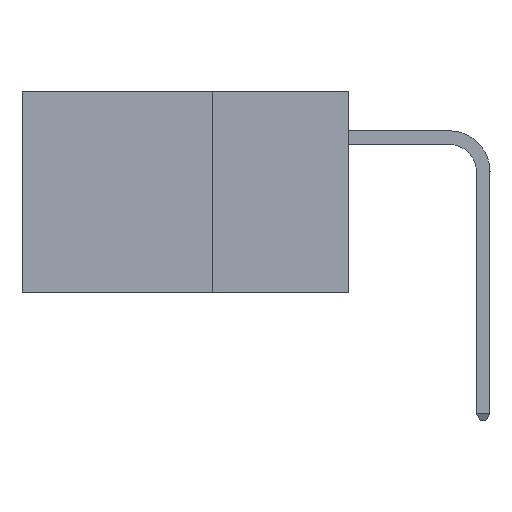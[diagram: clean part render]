
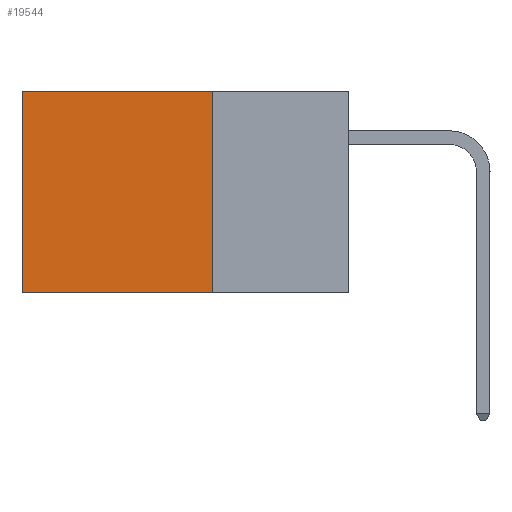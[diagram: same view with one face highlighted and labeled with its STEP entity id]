
A CAD part, left-side view. The second image highlights one B-rep face of the part: STEP entity #19544.
In plain terms, the highlighted planar face has unit normal (-1, 0, 0).
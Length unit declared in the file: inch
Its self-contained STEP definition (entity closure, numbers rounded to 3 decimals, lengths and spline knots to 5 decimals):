
#940 = VECTOR ( 'NONE', #22115, 39.37008 ) ;
#2225 = VERTEX_POINT ( 'NONE', #16818 ) ;
#3332 = VERTEX_POINT ( 'NONE', #12227 ) ;
#3860 = EDGE_CURVE ( 'NONE', #16594, #2225, #22168, .T. ) ;
#4036 = EDGE_CURVE ( 'NONE', #17334, #16594, #18546, .T. ) ;
#5055 = DIRECTION ( 'NONE',  ( 0., 1., 0. ) ) ;
#5182 = EDGE_LOOP ( 'NONE', ( #22476, #19031, #19371, #11590 ) ) ;
#6931 = CARTESIAN_POINT ( 'NONE',  ( 0.2875, 0.25, 0. ) ) ;
#7536 = VECTOR ( 'NONE', #5055, 39.37008 ) ;
#7874 = EDGE_CURVE ( 'NONE', #17334, #3332, #16626, .T. ) ;
#8077 = DIRECTION ( 'NONE',  ( 1., 0., 0. ) ) ;
#9849 = CARTESIAN_POINT ( 'NONE',  ( 0.2875, 0.25, 0. ) ) ;
#10452 = CARTESIAN_POINT ( 'NONE',  ( 0.2875, 0.25, 0. ) ) ;
#11590 = ORIENTED_EDGE ( 'NONE', *, *, #4036, .T. ) ;
#12227 = CARTESIAN_POINT ( 'NONE',  ( 0.2875, 0.25, -0.37 ) ) ;
#12296 = DIRECTION ( 'NONE',  ( 0., 0., -1. ) ) ;
#12707 = FACE_OUTER_BOUND ( 'NONE', #5182, .T. ) ;
#13000 = EDGE_CURVE ( 'NONE', #3332, #2225, #24052, .T. ) ;
#13105 = CARTESIAN_POINT ( 'NONE',  ( 0.2875, 0.25, -0.37 ) ) ;
#14227 = VECTOR ( 'NONE', #12296, 39.37008 ) ;
#16594 = VERTEX_POINT ( 'NONE', #24440 ) ;
#16626 = LINE ( 'NONE', #10452, #940 ) ;
#16818 = CARTESIAN_POINT ( 'NONE',  ( 0.2875, 0.6, -0.37 ) ) ;
#17334 = VERTEX_POINT ( 'NONE', #20682 ) ;
#17964 = AXIS2_PLACEMENT_3D ( 'NONE', #9849, #8077, #21690 ) ;
#18546 = LINE ( 'NONE', #6931, #7536 ) ;
#19031 = ORIENTED_EDGE ( 'NONE', *, *, #13000, .F. ) ;
#19371 = ORIENTED_EDGE ( 'NONE', *, *, #7874, .F. ) ;
#19544 = ADVANCED_FACE ( 'NONE', ( #12707 ), #19750, .F. ) ;
#19750 = PLANE ( 'NONE',  #17964 ) ;
#20682 = CARTESIAN_POINT ( 'NONE',  ( 0.2875, 0.25, 0. ) ) ;
#20888 = DIRECTION ( 'NONE',  ( 0., 1., 0. ) ) ;
#21690 = DIRECTION ( 'NONE',  ( 0., 0., -1. ) ) ;
#22115 = DIRECTION ( 'NONE',  ( 0., 0., -1. ) ) ;
#22168 = LINE ( 'NONE', #24032, #14227 ) ;
#22476 = ORIENTED_EDGE ( 'NONE', *, *, #3860, .T. ) ;
#24032 = CARTESIAN_POINT ( 'NONE',  ( 0.2875, 0.6, 0. ) ) ;
#24052 = LINE ( 'NONE', #13105, #25277 ) ;
#24440 = CARTESIAN_POINT ( 'NONE',  ( 0.2875, 0.6, 0. ) ) ;
#25277 = VECTOR ( 'NONE', #20888, 39.37008 ) ;
